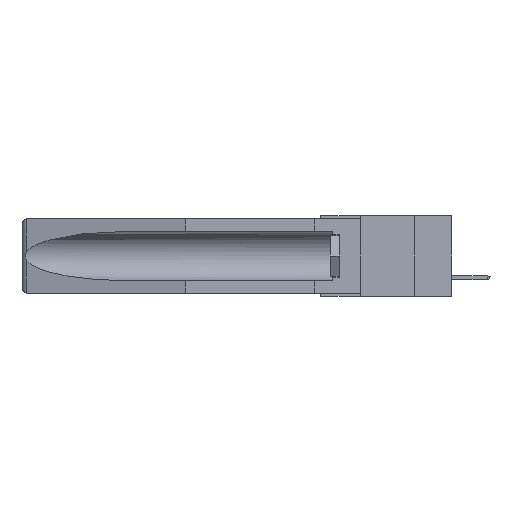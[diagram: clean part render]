
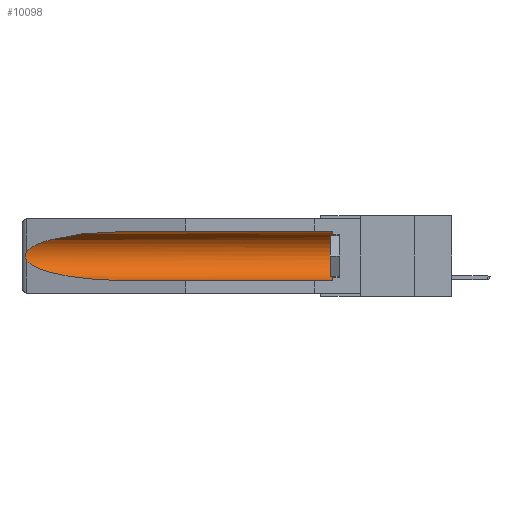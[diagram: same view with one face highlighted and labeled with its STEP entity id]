
A CAD part, left-side view. The second image highlights one B-rep face of the part: STEP entity #10098.
In plain terms, the highlighted cylindrical face has radius 2.857 mm (diameter 5.715 mm), a partial arc.
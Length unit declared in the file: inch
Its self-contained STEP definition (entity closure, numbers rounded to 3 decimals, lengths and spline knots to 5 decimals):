
#395 = VERTEX_POINT ( 'NONE', #13214 ) ;
#642 = EDGE_LOOP ( 'NONE', ( #5313, #1460, #8296, #3497, #7611, #11522 ) ) ;
#644 = CARTESIAN_POINT ( 'NONE',  ( 0.26597, 1.52961, -0.15275 ) ) ;
#715 = FACE_OUTER_BOUND ( 'NONE', #642, .T. ) ;
#1460 = ORIENTED_EDGE ( 'NONE', *, *, #5239, .T. ) ;
#1547 = CARTESIAN_POINT ( 'NONE',  ( 0.25451, 1.48313, -0.24835 ) ) ;
#2287 = DIRECTION ( 'NONE',  ( 0., 0., 1. ) ) ;
#2370 = CARTESIAN_POINT ( 'NONE',  ( 0.2673, 1.5327, -0.16383 ) ) ;
#3173 = VERTEX_POINT ( 'NONE', #5143 ) ;
#3497 = ORIENTED_EDGE ( 'NONE', *, *, #7396, .F. ) ;
#4379 =( BOUNDED_CURVE ( )  B_SPLINE_CURVE ( 3, ( #4738, #1547, #12874, #11329 ),
 .UNSPECIFIED., .F., .T. ) 
 B_SPLINE_CURVE_WITH_KNOTS ( ( 4, 4 ),
 ( 0.1948, 1.5708 ),
 .UNSPECIFIED. ) 
 CURVE ( )  GEOMETRIC_REPRESENTATION_ITEM ( )  RATIONAL_B_SPLINE_CURVE ( ( 1., 0.848, 0.848, 1. ) ) 
 REPRESENTATION_ITEM ( '' )  );
#4738 = CARTESIAN_POINT ( 'NONE',  ( 0.26537, 1.52718, -0.19328 ) ) ;
#5032 = CIRCLE ( 'NONE', #20559, 0.1125 ) ;
#5143 = CARTESIAN_POINT ( 'NONE',  ( 0.155, 1.07973, -0.284 ) ) ;
#5239 = EDGE_CURVE ( 'NONE', #20224, #395, #11266, .T. ) ;
#5313 = ORIENTED_EDGE ( 'NONE', *, *, #16363, .T. ) ;
#5391 = CARTESIAN_POINT ( 'NONE',  ( 0.21114, 1.30732, -0.059 ) ) ;
#5466 = CARTESIAN_POINT ( 'NONE',  ( 0.155, 0.126, -0.284 ) ) ;
#5962 = CARTESIAN_POINT ( 'NONE',  ( 0.26655, 1.53094, -0.18657 ) ) ;
#6023 = CARTESIAN_POINT ( 'NONE',  ( 0.26537, 1.52718, -0.19328 ) ) ;
#6163 = DIRECTION ( 'NONE',  ( 0., 1., 0. ) ) ;
#6947 = DIRECTION ( 'NONE',  ( 0., 1., 0. ) ) ;
#6948 = CARTESIAN_POINT ( 'NONE',  ( 0.155, 1.07973, -0.059 ) ) ;
#7034 = LINE ( 'NONE', #16705, #8277 ) ;
#7230 = CARTESIAN_POINT ( 'NONE',  ( 0.2675, 1.53308, -0.17534 ) ) ;
#7396 = EDGE_CURVE ( 'NONE', #12918, #3173, #7986, .T. ) ;
#7611 = ORIENTED_EDGE ( 'NONE', *, *, #10123, .T. ) ;
#7986 = LINE ( 'NONE', #7999, #19407 ) ;
#7999 = CARTESIAN_POINT ( 'NONE',  ( 0.155, -0.30754, -0.284 ) ) ;
#8277 = VECTOR ( 'NONE', #18062, 39.37008 ) ;
#8296 = ORIENTED_EDGE ( 'NONE', *, *, #11892, .T. ) ;
#8560 = CYLINDRICAL_SURFACE ( 'NONE', #11509, 0.1125 ) ;
#8699 = CARTESIAN_POINT ( 'NONE',  ( 0.25451, 1.48313, -0.09465 ) ) ;
#10098 = ADVANCED_FACE ( 'NONE', ( #715 ), #8560, .F. ) ;
#10123 = EDGE_CURVE ( 'NONE', #12918, #12289, #5032, .T. ) ;
#10510 = CARTESIAN_POINT ( 'NONE',  ( 0.2673, 1.53269, -0.17917 ) ) ;
#10780 = EDGE_CURVE ( 'NONE', #12289, #16586, #7034, .T. ) ;
#11266 = B_SPLINE_CURVE_WITH_KNOTS ( 'NONE', 3,
 ( #20180, #644, #15436, #2370, #16929, #7230, #10510, #5962, #12553, #6023 ),
 .UNSPECIFIED., .F., .F.,
 ( 4, 2, 2, 2, 4 ),
 ( 0., 0.00029, 0.00058, 0.00087, 0.00117 ),
 .UNSPECIFIED. ) ;
#11329 = CARTESIAN_POINT ( 'NONE',  ( 0.155, 1.07973, -0.284 ) ) ;
#11509 = AXIS2_PLACEMENT_3D ( 'NONE', #14932, #6947, #2287 ) ;
#11522 = ORIENTED_EDGE ( 'NONE', *, *, #10780, .T. ) ;
#11892 = EDGE_CURVE ( 'NONE', #395, #3173, #4379, .T. ) ;
#12289 = VERTEX_POINT ( 'NONE', #15170 ) ;
#12553 = CARTESIAN_POINT ( 'NONE',  ( 0.26597, 1.5296, -0.19026 ) ) ;
#12807 =( BOUNDED_CURVE ( )  B_SPLINE_CURVE ( 3, ( #6948, #5391, #8699, #14860 ),
 .UNSPECIFIED., .F., .F. ) 
 B_SPLINE_CURVE_WITH_KNOTS ( ( 4, 4 ),
 ( 4.71239, 6.08839 ),
 .UNSPECIFIED. ) 
 CURVE ( )  GEOMETRIC_REPRESENTATION_ITEM ( )  RATIONAL_B_SPLINE_CURVE ( ( 1., 0.848, 0.848, 1. ) ) 
 REPRESENTATION_ITEM ( '' )  );
#12874 = CARTESIAN_POINT ( 'NONE',  ( 0.21114, 1.30732, -0.284 ) ) ;
#12918 = VERTEX_POINT ( 'NONE', #5466 ) ;
#13214 = CARTESIAN_POINT ( 'NONE',  ( 0.26537, 1.52718, -0.19328 ) ) ;
#14860 = CARTESIAN_POINT ( 'NONE',  ( 0.26537, 1.52718, -0.14972 ) ) ;
#14932 = CARTESIAN_POINT ( 'NONE',  ( 0.155, -0.30754, -0.1715 ) ) ;
#15170 = CARTESIAN_POINT ( 'NONE',  ( 0.155, 0.126, -0.059 ) ) ;
#15436 = CARTESIAN_POINT ( 'NONE',  ( 0.26654, 1.53092, -0.15636 ) ) ;
#16231 = CARTESIAN_POINT ( 'NONE',  ( 0.26537, 1.52718, -0.14972 ) ) ;
#16363 = EDGE_CURVE ( 'NONE', #16586, #20224, #12807, .T. ) ;
#16586 = VERTEX_POINT ( 'NONE', #20725 ) ;
#16705 = CARTESIAN_POINT ( 'NONE',  ( 0.155, -0.30754, -0.059 ) ) ;
#16929 = CARTESIAN_POINT ( 'NONE',  ( 0.2675, 1.53308, -0.16763 ) ) ;
#17125 = DIRECTION ( 'NONE',  ( 0., -1., 0. ) ) ;
#18062 = DIRECTION ( 'NONE',  ( 0., 1., 0. ) ) ;
#18705 = DIRECTION ( 'NONE',  ( 0., 0., 1. ) ) ;
#19407 = VECTOR ( 'NONE', #6163, 39.37008 ) ;
#20180 = CARTESIAN_POINT ( 'NONE',  ( 0.26537, 1.52718, -0.14972 ) ) ;
#20224 = VERTEX_POINT ( 'NONE', #16231 ) ;
#20295 = CARTESIAN_POINT ( 'NONE',  ( 0.155, 0.126, -0.1715 ) ) ;
#20559 = AXIS2_PLACEMENT_3D ( 'NONE', #20295, #17125, #18705 ) ;
#20725 = CARTESIAN_POINT ( 'NONE',  ( 0.155, 1.07973, -0.059 ) ) ;
